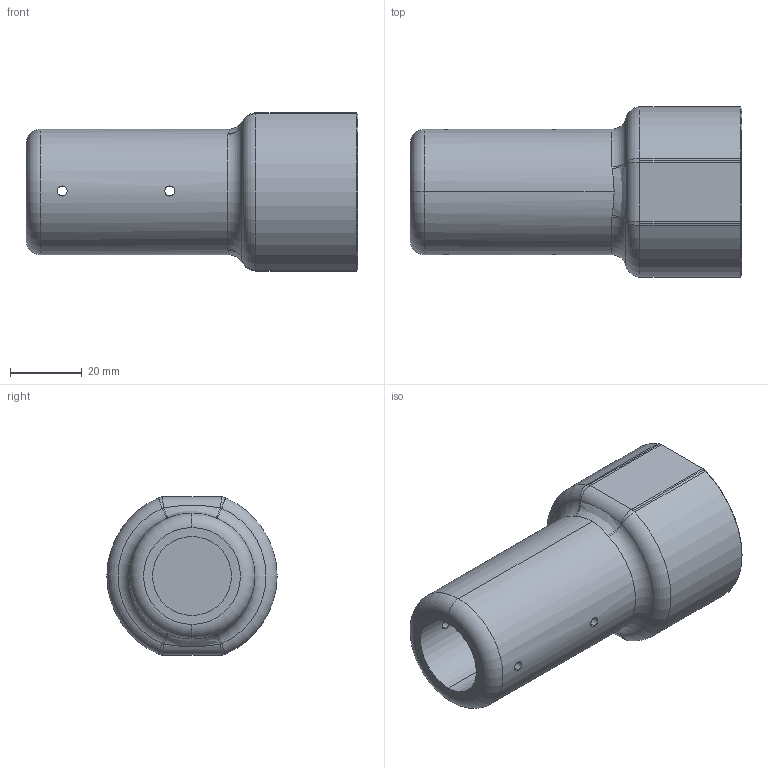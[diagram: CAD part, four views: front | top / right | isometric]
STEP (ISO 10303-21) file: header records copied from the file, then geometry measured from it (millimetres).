
FILE_DESCRIPTION (( 'STEP AP203' ), '1' );
FILE_NAME ('MOD9_PVC_stock_adapter.STEP', '2020-07-17T22:53:37', ( '' ), ( '' ), 'SwSTEP 2.0', 'SolidWorks 2019', '' );
FILE_SCHEMA (( 'CONFIG_CONTROL_DESIGN' ));
Length unit declared in the file: millimetre
Products named in the file (1): MOD9_PVC_stock_adapter
Bounding box: 92.37 x 47.42 x 44.06 mm (x, y, z)
Volume: 75605 mm3; surface area: 21062.8 mm2
Topology: 1 solids, 1 shells, 94 faces, 216 edges, 126 vertices
Faces by surface type: cylinder 32, cone 26, plane 20, bspline 10, torus 6
Entity records: 3405 total; most frequent: CARTESIAN_POINT 1253, ORIENTED_EDGE 432, DIRECTION 432, EDGE_CURVE 216, AXIS2_PLACEMENT_3D 169, VERTEX_POINT 126, EDGE_LOOP 104, FACE_OUTER_BOUND 94
